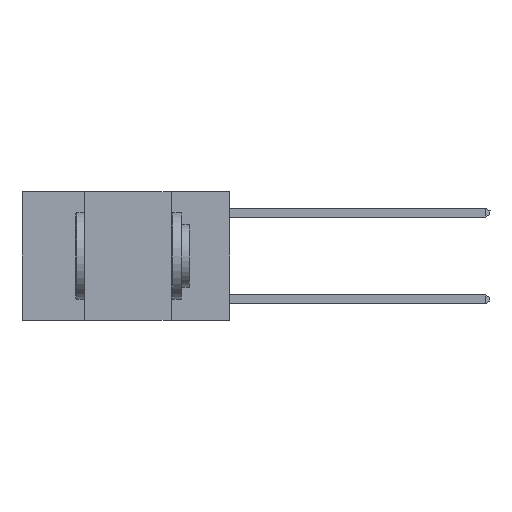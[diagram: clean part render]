
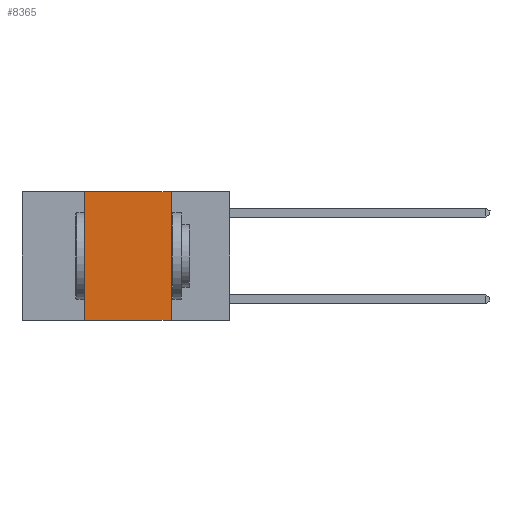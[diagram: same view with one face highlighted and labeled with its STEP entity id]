
A CAD part, left-side view. The second image highlights one B-rep face of the part: STEP entity #8365.
In plain terms, the highlighted planar face has unit normal (-1, 0, 0).
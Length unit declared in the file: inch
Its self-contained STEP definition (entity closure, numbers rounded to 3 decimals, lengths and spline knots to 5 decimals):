
#488 = LINE ( 'NONE', #11983, #6764 ) ;
#549 = DIRECTION ( 'NONE',  ( 0., -1., 0. ) ) ;
#862 = VECTOR ( 'NONE', #15721, 39.37008 ) ;
#1118 = DIRECTION ( 'NONE',  ( 0., 0., 1. ) ) ;
#1262 = EDGE_LOOP ( 'NONE', ( #6483, #1387, #6301, #12030 ) ) ;
#1387 = ORIENTED_EDGE ( 'NONE', *, *, #12664, .F. ) ;
#2704 = CARTESIAN_POINT ( 'NONE',  ( 0., 0.42, -0.37 ) ) ;
#4217 = LINE ( 'NONE', #7358, #862 ) ;
#4322 = CARTESIAN_POINT ( 'NONE',  ( 0., 0.42, 0. ) ) ;
#5709 = AXIS2_PLACEMENT_3D ( 'NONE', #15312, #15362, #8199 ) ;
#6301 = ORIENTED_EDGE ( 'NONE', *, *, #13250, .F. ) ;
#6483 = ORIENTED_EDGE ( 'NONE', *, *, #14031, .F. ) ;
#6586 = LINE ( 'NONE', #9197, #13767 ) ;
#6764 = VECTOR ( 'NONE', #13202, 39.37008 ) ;
#7358 = CARTESIAN_POINT ( 'NONE',  ( 0., 0.17, 0. ) ) ;
#8199 = DIRECTION ( 'NONE',  ( 0., 0., -1. ) ) ;
#8365 = ADVANCED_FACE ( 'NONE', ( #15613 ), #11836, .F. ) ;
#8973 = VERTEX_POINT ( 'NONE', #11612 ) ;
#9197 = CARTESIAN_POINT ( 'NONE',  ( 0., 0.6, -0.37 ) ) ;
#9857 = VERTEX_POINT ( 'NONE', #15674 ) ;
#10568 = VERTEX_POINT ( 'NONE', #15398 ) ;
#11612 = CARTESIAN_POINT ( 'NONE',  ( 0., 0.17, 0. ) ) ;
#11836 = PLANE ( 'NONE',  #5709 ) ;
#11983 = CARTESIAN_POINT ( 'NONE',  ( 0., 0.6, 0. ) ) ;
#12030 = ORIENTED_EDGE ( 'NONE', *, *, #12454, .T. ) ;
#12454 = EDGE_CURVE ( 'NONE', #14249, #9857, #6586, .T. ) ;
#12664 = EDGE_CURVE ( 'NONE', #10568, #8973, #488, .T. ) ;
#13202 = DIRECTION ( 'NONE',  ( 0., -1., 0. ) ) ;
#13250 = EDGE_CURVE ( 'NONE', #14249, #10568, #15024, .T. ) ;
#13767 = VECTOR ( 'NONE', #549, 39.37008 ) ;
#14031 = EDGE_CURVE ( 'NONE', #8973, #9857, #4217, .T. ) ;
#14249 = VERTEX_POINT ( 'NONE', #2704 ) ;
#14658 = VECTOR ( 'NONE', #1118, 39.37008 ) ;
#15024 = LINE ( 'NONE', #4322, #14658 ) ;
#15312 = CARTESIAN_POINT ( 'NONE',  ( 0., 0.6, 0. ) ) ;
#15362 = DIRECTION ( 'NONE',  ( 1., 0., 0. ) ) ;
#15398 = CARTESIAN_POINT ( 'NONE',  ( 0., 0.42, 0. ) ) ;
#15613 = FACE_OUTER_BOUND ( 'NONE', #1262, .T. ) ;
#15674 = CARTESIAN_POINT ( 'NONE',  ( 0., 0.17, -0.37 ) ) ;
#15721 = DIRECTION ( 'NONE',  ( 0., 0., -1. ) ) ;
